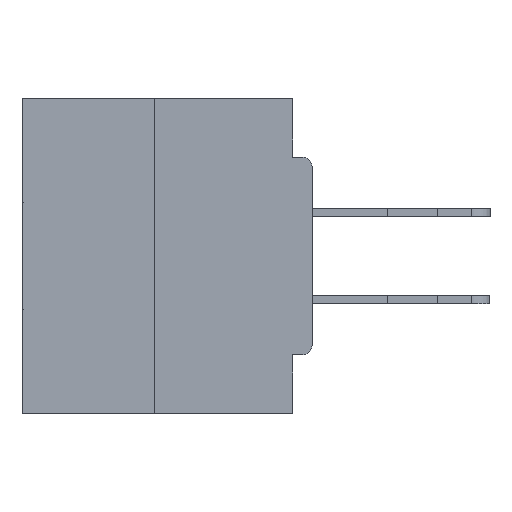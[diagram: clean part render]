
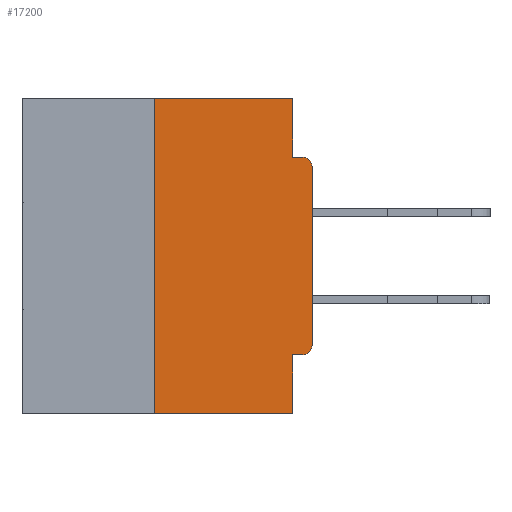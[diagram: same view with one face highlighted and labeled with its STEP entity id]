
A CAD part, left-side view. The second image highlights one B-rep face of the part: STEP entity #17200.
In plain terms, the highlighted planar face has unit normal (-1, 0, 0).
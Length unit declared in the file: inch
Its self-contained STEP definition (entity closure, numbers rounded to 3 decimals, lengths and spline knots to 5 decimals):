
#872 = DIRECTION ( 'NONE',  ( 0., 0., 1. ) ) ;
#1855 = VECTOR ( 'NONE', #872, 39.37008 ) ;
#1950 = DIRECTION ( 'NONE',  ( 0., 0., -1. ) ) ;
#2270 = VECTOR ( 'NONE', #13815, 39.37008 ) ;
#3318 = LINE ( 'NONE', #36843, #8278 ) ;
#4090 = LINE ( 'NONE', #27488, #5617 ) ;
#4177 = LINE ( 'NONE', #6959, #24423 ) ;
#4749 = LINE ( 'NONE', #39036, #2270 ) ;
#5066 = ORIENTED_EDGE ( 'NONE', *, *, #18953, .F. ) ;
#5159 = CARTESIAN_POINT ( 'NONE',  ( 0., 0.46, 0. ) ) ;
#5617 = VECTOR ( 'NONE', #30838, 39.37008 ) ;
#6959 = CARTESIAN_POINT ( 'NONE',  ( 0., 0.031, -0.5 ) ) ;
#7318 = CARTESIAN_POINT ( 'NONE',  ( 0., 0., -0.4065 ) ) ;
#7810 = CIRCLE ( 'NONE', #16445, 0.015 ) ;
#8204 = ORIENTED_EDGE ( 'NONE', *, *, #33606, .T. ) ;
#8278 = VECTOR ( 'NONE', #27683, 39.37008 ) ;
#8375 = DIRECTION ( 'NONE',  ( -1., 0., 0. ) ) ;
#8501 = ORIENTED_EDGE ( 'NONE', *, *, #30656, .F. ) ;
#8554 = VERTEX_POINT ( 'NONE', #28901 ) ;
#9158 = DIRECTION ( 'NONE',  ( -1., 0., 0. ) ) ;
#9739 = CARTESIAN_POINT ( 'NONE',  ( 0., 0.031, -0.0935 ) ) ;
#10404 = EDGE_LOOP ( 'NONE', ( #8501, #26932, #33751, #19933, #5066, #36689, #17351, #8204, #39249, #20774 ) ) ;
#10579 = VERTEX_POINT ( 'NONE', #22116 ) ;
#10750 = EDGE_CURVE ( 'NONE', #34540, #23675, #4749, .T. ) ;
#11389 = CARTESIAN_POINT ( 'NONE',  ( 0., 0.015, -0.4065 ) ) ;
#12504 = CIRCLE ( 'NONE', #19488, 0.015 ) ;
#13321 = DIRECTION ( 'NONE',  ( 0., 0., -1. ) ) ;
#13554 = CARTESIAN_POINT ( 'NONE',  ( 0., 0., -0.1085 ) ) ;
#13815 = DIRECTION ( 'NONE',  ( 0., -1., 0. ) ) ;
#14093 = LINE ( 'NONE', #35990, #32379 ) ;
#15007 = LINE ( 'NONE', #7318, #35297 ) ;
#15613 = VERTEX_POINT ( 'NONE', #26491 ) ;
#15762 = EDGE_CURVE ( 'NONE', #18255, #10579, #3318, .T. ) ;
#16445 = AXIS2_PLACEMENT_3D ( 'NONE', #40260, #8375, #39972 ) ;
#17200 = ADVANCED_FACE ( 'NONE', ( #23394 ), #17585, .F. ) ;
#17351 = ORIENTED_EDGE ( 'NONE', *, *, #32635, .T. ) ;
#17585 = PLANE ( 'NONE',  #36896 ) ;
#18255 = VERTEX_POINT ( 'NONE', #9739 ) ;
#18953 = EDGE_CURVE ( 'NONE', #22643, #15613, #15007, .T. ) ;
#19488 = AXIS2_PLACEMENT_3D ( 'NONE', #30690, #9158, #33750 ) ;
#19890 = CARTESIAN_POINT ( 'NONE',  ( 0., 0.25, 0. ) ) ;
#19933 = ORIENTED_EDGE ( 'NONE', *, *, #34661, .F. ) ;
#20774 = ORIENTED_EDGE ( 'NONE', *, *, #24387, .F. ) ;
#21283 = VERTEX_POINT ( 'NONE', #13554 ) ;
#22022 = VERTEX_POINT ( 'NONE', #22708 ) ;
#22116 = CARTESIAN_POINT ( 'NONE',  ( 0., 0.015, -0.0935 ) ) ;
#22643 = VERTEX_POINT ( 'NONE', #11389 ) ;
#22708 = CARTESIAN_POINT ( 'NONE',  ( 0., 0.25, 0. ) ) ;
#22888 = DIRECTION ( 'NONE',  ( 0., 1., 0. ) ) ;
#23394 = FACE_OUTER_BOUND ( 'NONE', #10404, .T. ) ;
#23618 = VERTEX_POINT ( 'NONE', #25991 ) ;
#23675 = VERTEX_POINT ( 'NONE', #35420 ) ;
#24387 = EDGE_CURVE ( 'NONE', #8554, #18255, #14093, .T. ) ;
#24423 = VECTOR ( 'NONE', #13321, 39.37008 ) ;
#25991 = CARTESIAN_POINT ( 'NONE',  ( 0., 0., -0.3915 ) ) ;
#26491 = CARTESIAN_POINT ( 'NONE',  ( 0., 0.031, -0.4065 ) ) ;
#26932 = ORIENTED_EDGE ( 'NONE', *, *, #39676, .F. ) ;
#27488 = CARTESIAN_POINT ( 'NONE',  ( 0., 0.46, 0. ) ) ;
#27683 = DIRECTION ( 'NONE',  ( 0., -1., 0. ) ) ;
#28901 = CARTESIAN_POINT ( 'NONE',  ( 0., 0.031, 0. ) ) ;
#30601 = EDGE_CURVE ( 'NONE', #22643, #23618, #12504, .T. ) ;
#30656 = EDGE_CURVE ( 'NONE', #22022, #8554, #4090, .T. ) ;
#30690 = CARTESIAN_POINT ( 'NONE',  ( 0., 0.015, -0.3915 ) ) ;
#30838 = DIRECTION ( 'NONE',  ( 0., -1., 0. ) ) ;
#32043 = LINE ( 'NONE', #19890, #1855 ) ;
#32379 = VECTOR ( 'NONE', #39106, 39.37008 ) ;
#32635 = EDGE_CURVE ( 'NONE', #23618, #21283, #36552, .T. ) ;
#33606 = EDGE_CURVE ( 'NONE', #21283, #10579, #7810, .T. ) ;
#33750 = DIRECTION ( 'NONE',  ( 0., 0., -1. ) ) ;
#33751 = ORIENTED_EDGE ( 'NONE', *, *, #10750, .T. ) ;
#34540 = VERTEX_POINT ( 'NONE', #40810 ) ;
#34661 = EDGE_CURVE ( 'NONE', #15613, #23675, #4177, .T. ) ;
#35099 = VECTOR ( 'NONE', #38283, 39.37008 ) ;
#35147 = CARTESIAN_POINT ( 'NONE',  ( 0., 0., 0. ) ) ;
#35297 = VECTOR ( 'NONE', #22888, 39.37008 ) ;
#35420 = CARTESIAN_POINT ( 'NONE',  ( 0., 0.031, -0.5 ) ) ;
#35990 = CARTESIAN_POINT ( 'NONE',  ( 0., 0.031, 0. ) ) ;
#36552 = LINE ( 'NONE', #35147, #35099 ) ;
#36689 = ORIENTED_EDGE ( 'NONE', *, *, #30601, .T. ) ;
#36843 = CARTESIAN_POINT ( 'NONE',  ( 0., 0., -0.0935 ) ) ;
#36896 = AXIS2_PLACEMENT_3D ( 'NONE', #5159, #39517, #1950 ) ;
#38283 = DIRECTION ( 'NONE',  ( 0., 0., 1. ) ) ;
#39036 = CARTESIAN_POINT ( 'NONE',  ( 0., 0.46, -0.5 ) ) ;
#39106 = DIRECTION ( 'NONE',  ( 0., 0., -1. ) ) ;
#39249 = ORIENTED_EDGE ( 'NONE', *, *, #15762, .F. ) ;
#39517 = DIRECTION ( 'NONE',  ( 1., 0., 0. ) ) ;
#39676 = EDGE_CURVE ( 'NONE', #34540, #22022, #32043, .T. ) ;
#39972 = DIRECTION ( 'NONE',  ( 0., 0., -1. ) ) ;
#40260 = CARTESIAN_POINT ( 'NONE',  ( 0., 0.015, -0.1085 ) ) ;
#40810 = CARTESIAN_POINT ( 'NONE',  ( 0., 0.25, -0.5 ) ) ;
